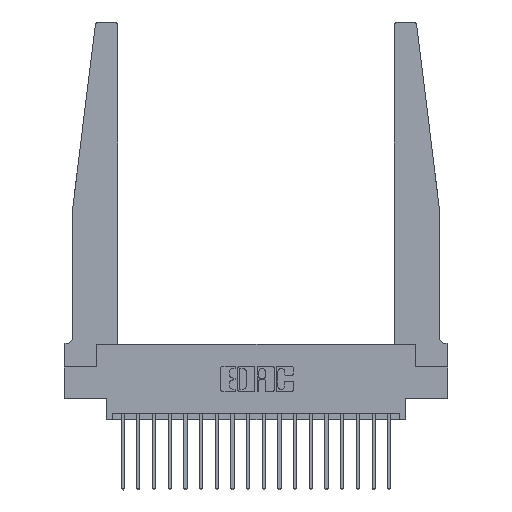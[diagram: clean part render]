
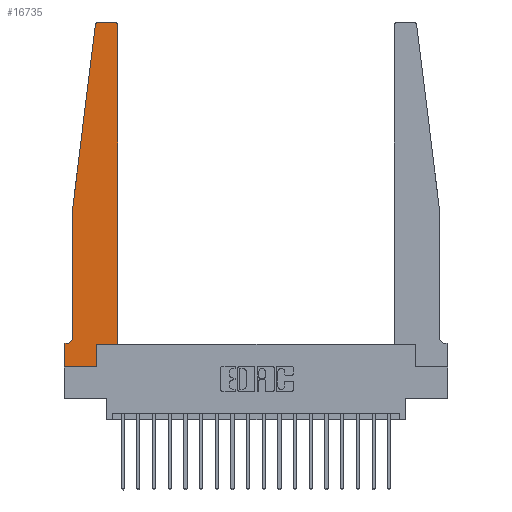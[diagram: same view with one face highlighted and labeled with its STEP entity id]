
A CAD part, top view. The second image highlights one B-rep face of the part: STEP entity #16735.
In plain terms, the highlighted planar face has unit normal (0, 0, 1).
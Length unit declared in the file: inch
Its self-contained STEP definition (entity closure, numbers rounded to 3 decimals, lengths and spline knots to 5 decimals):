
#28 = CARTESIAN_POINT ( 'NONE',  ( 0.065, 0.2375, 0.37 ) ) ;
#209 = VECTOR ( 'NONE', #5558, 39.37008 ) ;
#255 = DIRECTION ( 'NONE',  ( 0., 0., 1. ) ) ;
#342 = ORIENTED_EDGE ( 'NONE', *, *, #13658, .T. ) ;
#490 = VERTEX_POINT ( 'NONE', #9151 ) ;
#784 = ORIENTED_EDGE ( 'NONE', *, *, #19396, .T. ) ;
#859 = EDGE_LOOP ( 'NONE', ( #1711, #11519, #19278, #2249, #11129, #342, #3262, #18224, #784, #10496, #4557, #3219 ) ) ;
#1154 = CARTESIAN_POINT ( 'NONE',  ( 0.2605, 0., 0.37 ) ) ;
#1363 = LINE ( 'NONE', #9911, #5912 ) ;
#1499 = CARTESIAN_POINT ( 'NONE',  ( 0.015, 0.2375, 0.37 ) ) ;
#1519 = PLANE ( 'NONE',  #10634 ) ;
#1711 = ORIENTED_EDGE ( 'NONE', *, *, #18188, .T. ) ;
#1977 = VERTEX_POINT ( 'NONE', #14919 ) ;
#2249 = ORIENTED_EDGE ( 'NONE', *, *, #4186, .T. ) ;
#2308 = VECTOR ( 'NONE', #17203, 39.37008 ) ;
#2467 = VECTOR ( 'NONE', #12756, 39.37008 ) ;
#2516 = DIRECTION ( 'NONE',  ( 1., 0., 0. ) ) ;
#2672 = VECTOR ( 'NONE', #10529, 39.37008 ) ;
#2755 = AXIS2_PLACEMENT_3D ( 'NONE', #15946, #6705, #17494 ) ;
#2809 = DIRECTION ( 'NONE',  ( 0., 1., 0. ) ) ;
#2958 = LINE ( 'NONE', #3530, #2467 ) ;
#3045 = DIRECTION ( 'NONE',  ( -1., 0., 0. ) ) ;
#3086 = CARTESIAN_POINT ( 'NONE',  ( 0.2605, 0.18, 0.37 ) ) ;
#3219 = ORIENTED_EDGE ( 'NONE', *, *, #5355, .T. ) ;
#3262 = ORIENTED_EDGE ( 'NONE', *, *, #14993, .T. ) ;
#3295 = VERTEX_POINT ( 'NONE', #12199 ) ;
#3346 = VERTEX_POINT ( 'NONE', #28 ) ;
#3530 = CARTESIAN_POINT ( 'NONE',  ( 0.065, 1.25, 0.37 ) ) ;
#4029 = CARTESIAN_POINT ( 'NONE',  ( 0.065, 1.25, 0.37 ) ) ;
#4186 = EDGE_CURVE ( 'NONE', #5486, #3346, #12463, .T. ) ;
#4347 = CARTESIAN_POINT ( 'NONE',  ( 0.2605, 0.18, 0.37 ) ) ;
#4557 = ORIENTED_EDGE ( 'NONE', *, *, #4825, .T. ) ;
#4606 = CARTESIAN_POINT ( 'NONE',  ( 0., 0.1875, 0.37 ) ) ;
#4795 = CARTESIAN_POINT ( 'NONE',  ( 0.425, 0.18, 0.37 ) ) ;
#4825 = EDGE_CURVE ( 'NONE', #10136, #11698, #1363, .T. ) ;
#5355 = EDGE_CURVE ( 'NONE', #11698, #3295, #16741, .T. ) ;
#5486 = VERTEX_POINT ( 'NONE', #7113 ) ;
#5558 = DIRECTION ( 'NONE',  ( 0., -1., 0. ) ) ;
#5910 = VERTEX_POINT ( 'NONE', #19024 ) ;
#5912 = VECTOR ( 'NONE', #6800, 39.37008 ) ;
#6126 = CARTESIAN_POINT ( 'NONE',  ( 0.25, 2.75, 0.37 ) ) ;
#6140 = DIRECTION ( 'NONE',  ( 1., 0., 0. ) ) ;
#6338 = CARTESIAN_POINT ( 'NONE',  ( 0.24675, 2.72367, 0.37 ) ) ;
#6669 = DIRECTION ( 'NONE',  ( 0., -1., 0. ) ) ;
#6705 = DIRECTION ( 'NONE',  ( 0., 0., 1. ) ) ;
#6740 = LINE ( 'NONE', #12016, #2672 ) ;
#6800 = DIRECTION ( 'NONE',  ( 0., 1., 0. ) ) ;
#6865 = EDGE_CURVE ( 'NONE', #3346, #490, #12895, .T. ) ;
#7113 = CARTESIAN_POINT ( 'NONE',  ( 0.065, 1.25, 0.37 ) ) ;
#7542 = VECTOR ( 'NONE', #2809, 39.37008 ) ;
#7972 = CARTESIAN_POINT ( 'NONE',  ( 0.425, 0.18, 0.37 ) ) ;
#8292 = EDGE_CURVE ( 'NONE', #13276, #5486, #2958, .T. ) ;
#8408 = EDGE_CURVE ( 'NONE', #18568, #13276, #12338, .T. ) ;
#8577 = AXIS2_PLACEMENT_3D ( 'NONE', #9422, #255, #10993 ) ;
#8703 = CARTESIAN_POINT ( 'NONE',  ( 0.425, 2.72, 0.37 ) ) ;
#9151 = CARTESIAN_POINT ( 'NONE',  ( 0.015, 0.1875, 0.37 ) ) ;
#9320 = VERTEX_POINT ( 'NONE', #1154 ) ;
#9422 = CARTESIAN_POINT ( 'NONE',  ( 0.27653, 2.72, 0.37 ) ) ;
#9643 = EDGE_CURVE ( 'NONE', #16083, #10136, #10501, .T. ) ;
#9911 = CARTESIAN_POINT ( 'NONE',  ( 0.425, 0.18, 0.37 ) ) ;
#10136 = VERTEX_POINT ( 'NONE', #4795 ) ;
#10496 = ORIENTED_EDGE ( 'NONE', *, *, #9643, .T. ) ;
#10501 = LINE ( 'NONE', #7972, #2308 ) ;
#10529 = DIRECTION ( 'NONE',  ( -1., 0., 0. ) ) ;
#10634 = AXIS2_PLACEMENT_3D ( 'NONE', #4606, #15376, #6140 ) ;
#10805 = VECTOR ( 'NONE', #2516, 39.37008 ) ;
#10993 = DIRECTION ( 'NONE',  ( 1., 0., 0. ) ) ;
#11129 = ORIENTED_EDGE ( 'NONE', *, *, #6865, .T. ) ;
#11519 = ORIENTED_EDGE ( 'NONE', *, *, #8408, .T. ) ;
#11549 = AXIS2_PLACEMENT_3D ( 'NONE', #1499, #12271, #3045 ) ;
#11698 = VERTEX_POINT ( 'NONE', #8703 ) ;
#12016 = CARTESIAN_POINT ( 'NONE',  ( 0.065, 0.1875, 0.37 ) ) ;
#12199 = CARTESIAN_POINT ( 'NONE',  ( 0.395, 2.75, 0.37 ) ) ;
#12271 = DIRECTION ( 'NONE',  ( 0., 0., -1. ) ) ;
#12338 = CIRCLE ( 'NONE', #8577, 0.03 ) ;
#12463 = LINE ( 'NONE', #4029, #209 ) ;
#12756 = DIRECTION ( 'NONE',  ( -0.122, -0.992, 0. ) ) ;
#12895 = CIRCLE ( 'NONE', #11549, 0.05 ) ;
#13155 = CARTESIAN_POINT ( 'NONE',  ( 0.27653, 2.75, 0.37 ) ) ;
#13276 = VERTEX_POINT ( 'NONE', #6338 ) ;
#13302 = CARTESIAN_POINT ( 'NONE',  ( 0., 0., 0.37 ) ) ;
#13658 = EDGE_CURVE ( 'NONE', #490, #1977, #6740, .T. ) ;
#14919 = CARTESIAN_POINT ( 'NONE',  ( 0., 0.1875, 0.37 ) ) ;
#14993 = EDGE_CURVE ( 'NONE', #1977, #5910, #17793, .T. ) ;
#15144 = EDGE_CURVE ( 'NONE', #5910, #9320, #15368, .T. ) ;
#15269 = LINE ( 'NONE', #4347, #7542 ) ;
#15368 = LINE ( 'NONE', #13302, #10805 ) ;
#15376 = DIRECTION ( 'NONE',  ( 0., 0., 1. ) ) ;
#15545 = VECTOR ( 'NONE', #18460, 39.37008 ) ;
#15601 = FACE_OUTER_BOUND ( 'NONE', #859, .T. ) ;
#15946 = CARTESIAN_POINT ( 'NONE',  ( 0.395, 2.72, 0.37 ) ) ;
#15974 = CARTESIAN_POINT ( 'NONE',  ( 0., 0., 0.37 ) ) ;
#16032 = LINE ( 'NONE', #6126, #15545 ) ;
#16083 = VERTEX_POINT ( 'NONE', #3086 ) ;
#16735 = ADVANCED_FACE ( 'NONE', ( #15601 ), #1519, .T. ) ;
#16741 = CIRCLE ( 'NONE', #2755, 0.03 ) ;
#17203 = DIRECTION ( 'NONE',  ( 1., 0., 0. ) ) ;
#17295 = VECTOR ( 'NONE', #6669, 39.37008 ) ;
#17494 = DIRECTION ( 'NONE',  ( 1., 0., 0. ) ) ;
#17793 = LINE ( 'NONE', #15974, #17295 ) ;
#18188 = EDGE_CURVE ( 'NONE', #3295, #18568, #16032, .T. ) ;
#18224 = ORIENTED_EDGE ( 'NONE', *, *, #15144, .T. ) ;
#18460 = DIRECTION ( 'NONE',  ( -1., 0., 0. ) ) ;
#18568 = VERTEX_POINT ( 'NONE', #13155 ) ;
#19024 = CARTESIAN_POINT ( 'NONE',  ( 0., 0., 0.37 ) ) ;
#19278 = ORIENTED_EDGE ( 'NONE', *, *, #8292, .T. ) ;
#19396 = EDGE_CURVE ( 'NONE', #9320, #16083, #15269, .T. ) ;
